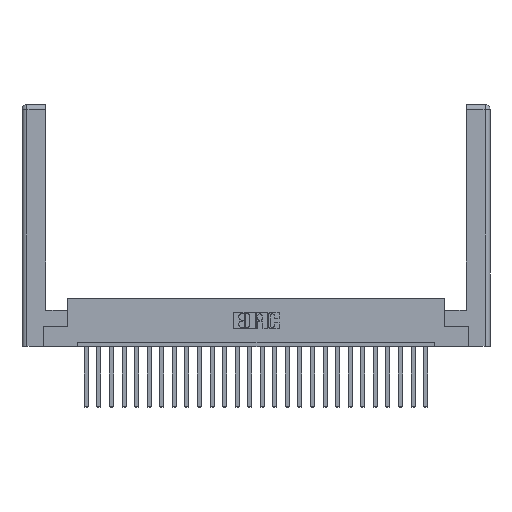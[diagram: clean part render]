
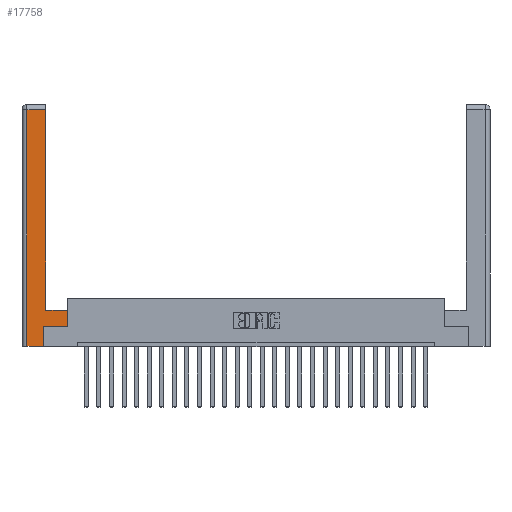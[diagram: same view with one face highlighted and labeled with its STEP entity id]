
A CAD part, top view. The second image highlights one B-rep face of the part: STEP entity #17758.
In plain terms, the highlighted planar face has unit normal (0, 0, 1).
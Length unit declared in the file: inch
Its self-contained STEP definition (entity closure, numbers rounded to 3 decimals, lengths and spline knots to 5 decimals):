
#127 = DIRECTION ( 'NONE',  ( -1., 0., 0. ) ) ;
#647 = FACE_OUTER_BOUND ( 'NONE', #8416, .T. ) ;
#954 = LINE ( 'NONE', #23380, #10715 ) ;
#988 = CARTESIAN_POINT ( 'NONE',  ( 0., 0., 0. ) ) ;
#1033 = AXIS2_PLACEMENT_3D ( 'NONE', #988, #16451, #5064 ) ;
#1555 = VECTOR ( 'NONE', #14409, 39.37008 ) ;
#2110 = DIRECTION ( 'NONE',  ( 0., 1., 0. ) ) ;
#2390 = ORIENTED_EDGE ( 'NONE', *, *, #5818, .T. ) ;
#2461 = CARTESIAN_POINT ( 'NONE',  ( 0.265, 0., 0. ) ) ;
#2742 = CARTESIAN_POINT ( 'NONE',  ( 0.0615, 2.94, 0. ) ) ;
#2812 = CARTESIAN_POINT ( 'NONE',  ( 0.265, 0.245, 0. ) ) ;
#3618 = DIRECTION ( 'NONE',  ( -1., 0., 0. ) ) ;
#3916 = EDGE_CURVE ( 'NONE', #6398, #13962, #10074, .T. ) ;
#4160 = CARTESIAN_POINT ( 'NONE',  ( 0.295, 3., 0. ) ) ;
#4520 = DIRECTION ( 'NONE',  ( 0., 1., 0. ) ) ;
#4837 = EDGE_CURVE ( 'NONE', #13962, #17481, #15335, .T. ) ;
#5064 = DIRECTION ( 'NONE',  ( -1., 0., 0. ) ) ;
#5257 = DIRECTION ( 'NONE',  ( 1., 0., 0. ) ) ;
#5818 = EDGE_CURVE ( 'NONE', #24418, #16942, #15312, .T. ) ;
#5891 = CARTESIAN_POINT ( 'NONE',  ( 0.0615, 2.94, 0. ) ) ;
#6180 = CARTESIAN_POINT ( 'NONE',  ( 0.295, 0.45, 0. ) ) ;
#6221 = VECTOR ( 'NONE', #9867, 39.37008 ) ;
#6398 = VERTEX_POINT ( 'NONE', #2742 ) ;
#6582 = VERTEX_POINT ( 'NONE', #21001 ) ;
#6631 = EDGE_CURVE ( 'NONE', #6582, #6811, #954, .T. ) ;
#6811 = VERTEX_POINT ( 'NONE', #17686 ) ;
#7490 = CARTESIAN_POINT ( 'NONE',  ( 0.295, 0.45, 0. ) ) ;
#7805 = CARTESIAN_POINT ( 'NONE',  ( 0.0615, 0., 0. ) ) ;
#8162 = LINE ( 'NONE', #11072, #24195 ) ;
#8324 = VECTOR ( 'NONE', #2110, 39.37008 ) ;
#8416 = EDGE_LOOP ( 'NONE', ( #2390, #23927, #12952, #23301, #11623, #10589, #19869, #15361 ) ) ;
#8748 = EDGE_CURVE ( 'NONE', #19857, #6582, #8162, .T. ) ;
#9146 = CARTESIAN_POINT ( 'NONE',  ( 0.265, 0.245, 0. ) ) ;
#9298 = VECTOR ( 'NONE', #127, 39.37008 ) ;
#9867 = DIRECTION ( 'NONE',  ( 1., 0., 0. ) ) ;
#10074 = LINE ( 'NONE', #12543, #1555 ) ;
#10589 = ORIENTED_EDGE ( 'NONE', *, *, #8748, .T. ) ;
#10715 = VECTOR ( 'NONE', #15594, 39.37008 ) ;
#11072 = CARTESIAN_POINT ( 'NONE',  ( 0.565, 0.245, 0. ) ) ;
#11623 = ORIENTED_EDGE ( 'NONE', *, *, #14278, .T. ) ;
#12543 = CARTESIAN_POINT ( 'NONE',  ( 0.0615, 0., 0. ) ) ;
#12646 = LINE ( 'NONE', #2812, #18058 ) ;
#12952 = ORIENTED_EDGE ( 'NONE', *, *, #3916, .T. ) ;
#13043 = EDGE_CURVE ( 'NONE', #6811, #24418, #16028, .T. ) ;
#13962 = VERTEX_POINT ( 'NONE', #7805 ) ;
#14278 = EDGE_CURVE ( 'NONE', #17481, #19857, #12646, .T. ) ;
#14409 = DIRECTION ( 'NONE',  ( 0., -1., 0. ) ) ;
#15312 = LINE ( 'NONE', #4160, #8324 ) ;
#15335 = LINE ( 'NONE', #21494, #6221 ) ;
#15361 = ORIENTED_EDGE ( 'NONE', *, *, #13043, .T. ) ;
#15594 = DIRECTION ( 'NONE',  ( 0., 1., 0. ) ) ;
#16028 = LINE ( 'NONE', #7490, #17844 ) ;
#16451 = DIRECTION ( 'NONE',  ( 0., 0., -1. ) ) ;
#16818 = CARTESIAN_POINT ( 'NONE',  ( 0.295, 2.94, 0. ) ) ;
#16942 = VERTEX_POINT ( 'NONE', #16818 ) ;
#17481 = VERTEX_POINT ( 'NONE', #2461 ) ;
#17686 = CARTESIAN_POINT ( 'NONE',  ( 0.565, 0.45, 0. ) ) ;
#17758 = ADVANCED_FACE ( 'NONE', ( #647 ), #24220, .F. ) ;
#17844 = VECTOR ( 'NONE', #3618, 39.37008 ) ;
#18058 = VECTOR ( 'NONE', #4520, 39.37008 ) ;
#19857 = VERTEX_POINT ( 'NONE', #9146 ) ;
#19869 = ORIENTED_EDGE ( 'NONE', *, *, #6631, .T. ) ;
#21001 = CARTESIAN_POINT ( 'NONE',  ( 0.565, 0.245, 0. ) ) ;
#21051 = EDGE_CURVE ( 'NONE', #16942, #6398, #22635, .T. ) ;
#21494 = CARTESIAN_POINT ( 'NONE',  ( 0.265, 0., 0. ) ) ;
#22635 = LINE ( 'NONE', #5891, #9298 ) ;
#23301 = ORIENTED_EDGE ( 'NONE', *, *, #4837, .T. ) ;
#23380 = CARTESIAN_POINT ( 'NONE',  ( 0.565, 0.45, 0. ) ) ;
#23927 = ORIENTED_EDGE ( 'NONE', *, *, #21051, .T. ) ;
#24195 = VECTOR ( 'NONE', #5257, 39.37008 ) ;
#24220 = PLANE ( 'NONE',  #1033 ) ;
#24418 = VERTEX_POINT ( 'NONE', #6180 ) ;
